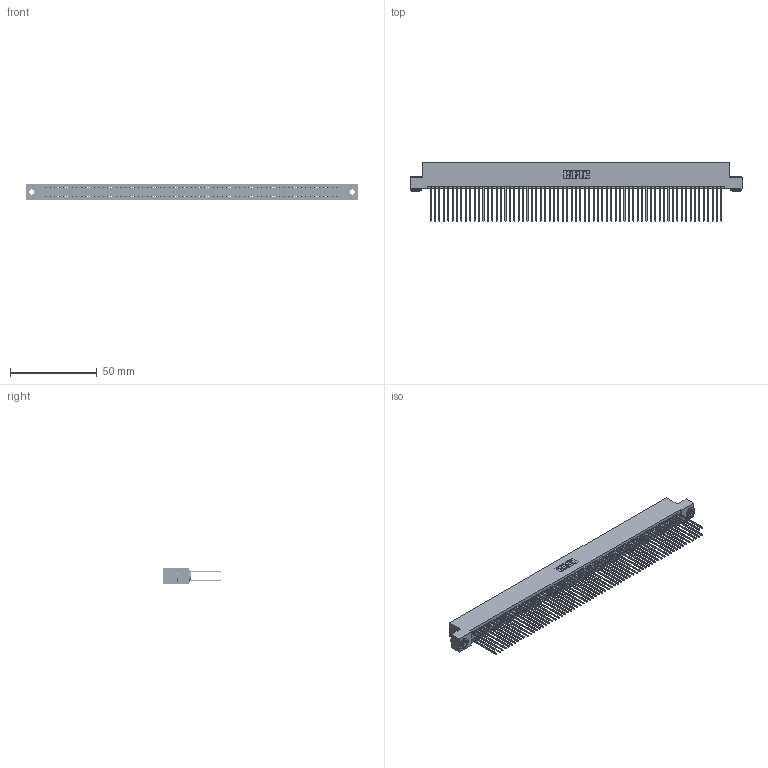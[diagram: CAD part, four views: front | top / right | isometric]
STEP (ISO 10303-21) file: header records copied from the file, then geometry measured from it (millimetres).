
FILE_DESCRIPTION (( 'STEP AP203' ), '1' );
FILE_NAME ('395-134-541-203.STEP', '2018-12-05T03:06:58', ( '' ), ( '' ), 'SwSTEP 2.0', 'SolidWorks 2016', '' );
FILE_SCHEMA (( 'CONFIG_CONTROL_DESIGN' ));
Length unit declared in the file: inch
Products named in the file (4): 345 Part_Flush Mounting Lugs - 0.156 Dia-TH; 345-292-001_345-293-141; 395-134-541-203; 345-250-002_345-250-002-102
Assembly tree (137 placements, depth 2):
  395-134-541-203
    345 Part_Flush Mounting Lugs - 0.156 Dia-TH
    345-292-001_345-293-141  x134
    345-250-002_345-250-002-102  x2
Bounding box: 191.39 x 33.96 x 9.4 mm (x, y, z)
Volume: 19611.9 mm3; surface area: 33292.7 mm2
Topology: 137 solids, 137 shells, 6864 faces, 20383 edges, 13406 vertices
Faces by surface type: plane 4512, cylinder 2344, cone 8
Entity records: 49872 total; most frequent: CARTESIAN_POINT 8311, ORIENTED_EDGE 8238, DIRECTION 7329, EDGE_CURVE 4119, LINE 3695, VECTOR 3695, VERTEX_POINT 2742, AXIS2_PLACEMENT_3D 1817
